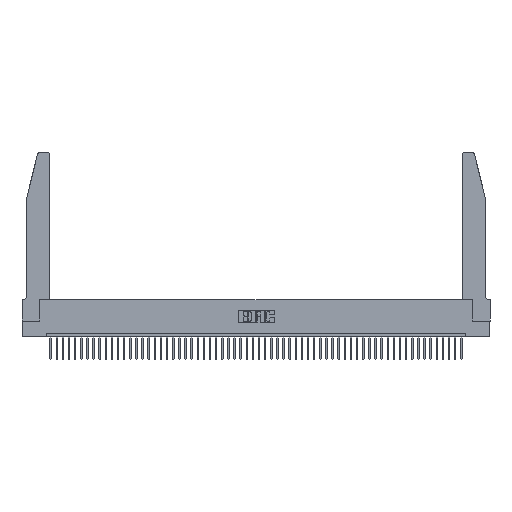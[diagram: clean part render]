
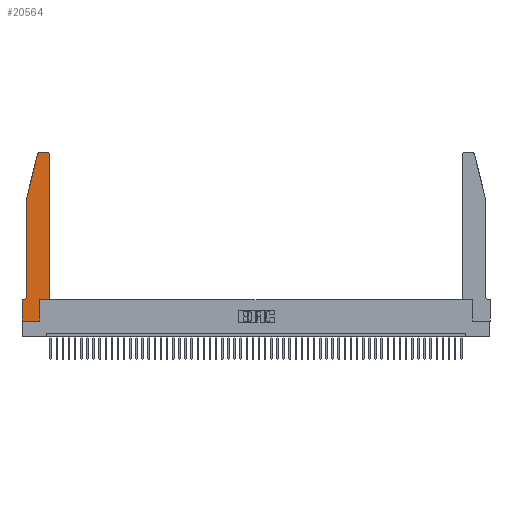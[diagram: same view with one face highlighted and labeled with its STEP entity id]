
A CAD part, top view. The second image highlights one B-rep face of the part: STEP entity #20564.
In plain terms, the highlighted planar face has unit normal (0, 0, 1).
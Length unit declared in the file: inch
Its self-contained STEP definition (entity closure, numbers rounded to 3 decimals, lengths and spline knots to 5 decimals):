
#170 = ORIENTED_EDGE ( 'NONE', *, *, #27050, .T. ) ;
#557 = CARTESIAN_POINT ( 'NONE',  ( 0.0055, 0.35, 0.37 ) ) ;
#560 = CARTESIAN_POINT ( 'NONE',  ( 0.4205, 2.75, 0.37 ) ) ;
#763 = VERTEX_POINT ( 'NONE', #13479 ) ;
#1389 = ORIENTED_EDGE ( 'NONE', *, *, #11748, .T. ) ;
#1840 = CARTESIAN_POINT ( 'NONE',  ( 0.0755, 2., 0.37 ) ) ;
#1872 = AXIS2_PLACEMENT_3D ( 'NONE', #17325, #6402, #38655 ) ;
#2724 = CARTESIAN_POINT ( 'NONE',  ( 0.0755, 0.42, 0.37 ) ) ;
#3187 = EDGE_CURVE ( 'NONE', #4844, #763, #23537, .T. ) ;
#3278 = EDGE_CURVE ( 'NONE', #38453, #35055, #41230, .T. ) ;
#4373 = VECTOR ( 'NONE', #25429, 39.37008 ) ;
#4844 = VERTEX_POINT ( 'NONE', #46409 ) ;
#5905 = DIRECTION ( 'NONE',  ( 0., 1., 0. ) ) ;
#6402 = DIRECTION ( 'NONE',  ( 0., 0., 1. ) ) ;
#6457 = VERTEX_POINT ( 'NONE', #557 ) ;
#6650 = LINE ( 'NONE', #36080, #19317 ) ;
#7045 = ORIENTED_EDGE ( 'NONE', *, *, #33911, .T. ) ;
#7117 = AXIS2_PLACEMENT_3D ( 'NONE', #15152, #44223, #43885 ) ;
#7120 = CARTESIAN_POINT ( 'NONE',  ( 0.2865, 0., 0.37 ) ) ;
#7476 = CARTESIAN_POINT ( 'NONE',  ( 0., 0., 0.37 ) ) ;
#8250 = LINE ( 'NONE', #39010, #17098 ) ;
#10651 = DIRECTION ( 'NONE',  ( 0., 1., 0. ) ) ;
#11029 = FACE_OUTER_BOUND ( 'NONE', #47378, .T. ) ;
#11257 = ORIENTED_EDGE ( 'NONE', *, *, #38534, .T. ) ;
#11748 = EDGE_CURVE ( 'NONE', #33758, #38453, #42578, .T. ) ;
#11949 = EDGE_CURVE ( 'NONE', #34345, #6457, #14689, .T. ) ;
#12480 = VERTEX_POINT ( 'NONE', #27450 ) ;
#12780 = LINE ( 'NONE', #49734, #30605 ) ;
#12926 = CARTESIAN_POINT ( 'NONE',  ( 0., 0., 0.37 ) ) ;
#13479 = CARTESIAN_POINT ( 'NONE',  ( 0.4505, 2.72, 0.37 ) ) ;
#13631 = VERTEX_POINT ( 'NONE', #42539 ) ;
#14689 = CIRCLE ( 'NONE', #44519, 0.07 ) ;
#15152 = CARTESIAN_POINT ( 'NONE',  ( 0., 0.35, 0.37 ) ) ;
#17098 = VECTOR ( 'NONE', #39556, 39.37008 ) ;
#17325 = CARTESIAN_POINT ( 'NONE',  ( 0.4205, 2.72, 0.37 ) ) ;
#17764 = CARTESIAN_POINT ( 'NONE',  ( 0.0755, 2., 0.37 ) ) ;
#19317 = VECTOR ( 'NONE', #28250, 39.37008 ) ;
#19671 = ORIENTED_EDGE ( 'NONE', *, *, #51198, .T. ) ;
#20564 = ADVANCED_FACE ( 'NONE', ( #11029 ), #27948, .T. ) ;
#22238 = CARTESIAN_POINT ( 'NONE',  ( 0.0755, 0.35, 0.37 ) ) ;
#22789 = ORIENTED_EDGE ( 'NONE', *, *, #3187, .T. ) ;
#23047 = VERTEX_POINT ( 'NONE', #48972 ) ;
#23537 = LINE ( 'NONE', #29133, #27998 ) ;
#23598 = DIRECTION ( 'NONE',  ( 1., 0., 0. ) ) ;
#25429 = DIRECTION ( 'NONE',  ( 0., -1., 0. ) ) ;
#25576 = CARTESIAN_POINT ( 'NONE',  ( 0., 0., 0.37 ) ) ;
#27050 = EDGE_CURVE ( 'NONE', #35055, #23047, #12780, .T. ) ;
#27436 = ORIENTED_EDGE ( 'NONE', *, *, #34682, .T. ) ;
#27450 = CARTESIAN_POINT ( 'NONE',  ( 0.284, 2.75, 0.37 ) ) ;
#27508 = CARTESIAN_POINT ( 'NONE',  ( 0.4505, 0.35, 0.37 ) ) ;
#27948 = PLANE ( 'NONE',  #7117 ) ;
#27998 = VECTOR ( 'NONE', #5905, 39.37008 ) ;
#28250 = DIRECTION ( 'NONE',  ( -0.239, -0.971, 0. ) ) ;
#29003 = LINE ( 'NONE', #22238, #30946 ) ;
#29133 = CARTESIAN_POINT ( 'NONE',  ( 0.4505, 0.35, 0.37 ) ) ;
#29560 = EDGE_CURVE ( 'NONE', #763, #35535, #46069, .T. ) ;
#30605 = VECTOR ( 'NONE', #10651, 39.37008 ) ;
#30667 = CARTESIAN_POINT ( 'NONE',  ( 0.0055, 0.42, 0.37 ) ) ;
#30946 = VECTOR ( 'NONE', #38593, 39.37008 ) ;
#32921 = CARTESIAN_POINT ( 'NONE',  ( 0., 0.35, 0.37 ) ) ;
#33758 = VERTEX_POINT ( 'NONE', #32921 ) ;
#33821 = ORIENTED_EDGE ( 'NONE', *, *, #36858, .T. ) ;
#33911 = EDGE_CURVE ( 'NONE', #23047, #4844, #50142, .T. ) ;
#34345 = VERTEX_POINT ( 'NONE', #2724 ) ;
#34682 = EDGE_CURVE ( 'NONE', #35535, #12480, #8250, .T. ) ;
#34852 = ORIENTED_EDGE ( 'NONE', *, *, #29560, .T. ) ;
#35055 = VERTEX_POINT ( 'NONE', #7120 ) ;
#35426 = EDGE_CURVE ( 'NONE', #35568, #34345, #36166, .T. ) ;
#35535 = VERTEX_POINT ( 'NONE', #560 ) ;
#35568 = VERTEX_POINT ( 'NONE', #1840 ) ;
#36080 = CARTESIAN_POINT ( 'NONE',  ( 0.0755, 2., 0.37 ) ) ;
#36166 = LINE ( 'NONE', #17764, #4373 ) ;
#36858 = EDGE_CURVE ( 'NONE', #13631, #35568, #6650, .T. ) ;
#37068 = ORIENTED_EDGE ( 'NONE', *, *, #35426, .T. ) ;
#37773 = ORIENTED_EDGE ( 'NONE', *, *, #3278, .T. ) ;
#38162 = VECTOR ( 'NONE', #39723, 39.37008 ) ;
#38453 = VERTEX_POINT ( 'NONE', #12926 ) ;
#38534 = EDGE_CURVE ( 'NONE', #12480, #13631, #47689, .T. ) ;
#38593 = DIRECTION ( 'NONE',  ( -1., 0., 0. ) ) ;
#38655 = DIRECTION ( 'NONE',  ( 1., 0., 0. ) ) ;
#38812 = DIRECTION ( 'NONE',  ( -1., 0., 0. ) ) ;
#39010 = CARTESIAN_POINT ( 'NONE',  ( 0.2605, 2.75, 0.37 ) ) ;
#39425 = DIRECTION ( 'NONE',  ( 1., 0., 0. ) ) ;
#39556 = DIRECTION ( 'NONE',  ( -1., 0., 0. ) ) ;
#39723 = DIRECTION ( 'NONE',  ( 1., 0., 0. ) ) ;
#40113 = CARTESIAN_POINT ( 'NONE',  ( 0.284, 2.72, 0.37 ) ) ;
#41230 = LINE ( 'NONE', #7476, #46287 ) ;
#42539 = CARTESIAN_POINT ( 'NONE',  ( 0.25487, 2.72718, 0.37 ) ) ;
#42578 = LINE ( 'NONE', #25576, #51478 ) ;
#43057 = DIRECTION ( 'NONE',  ( 0., 0., -1. ) ) ;
#43885 = DIRECTION ( 'NONE',  ( 1., 0., 0. ) ) ;
#44223 = DIRECTION ( 'NONE',  ( 0., 0., 1. ) ) ;
#44519 = AXIS2_PLACEMENT_3D ( 'NONE', #30667, #43057, #38812 ) ;
#45919 = AXIS2_PLACEMENT_3D ( 'NONE', #40113, #51629, #39425 ) ;
#46069 = CIRCLE ( 'NONE', #1872, 0.03 ) ;
#46287 = VECTOR ( 'NONE', #23598, 39.37008 ) ;
#46409 = CARTESIAN_POINT ( 'NONE',  ( 0.4505, 0.35, 0.37 ) ) ;
#47378 = EDGE_LOOP ( 'NONE', ( #27436, #11257, #33821, #37068, #50112, #19671, #1389, #37773, #170, #7045, #22789, #34852 ) ) ;
#47689 = CIRCLE ( 'NONE', #45919, 0.03 ) ;
#48972 = CARTESIAN_POINT ( 'NONE',  ( 0.2865, 0.35, 0.37 ) ) ;
#49734 = CARTESIAN_POINT ( 'NONE',  ( 0.2865, 0.35, 0.37 ) ) ;
#50112 = ORIENTED_EDGE ( 'NONE', *, *, #11949, .T. ) ;
#50142 = LINE ( 'NONE', #27508, #38162 ) ;
#50159 = DIRECTION ( 'NONE',  ( 0., -1., 0. ) ) ;
#51198 = EDGE_CURVE ( 'NONE', #6457, #33758, #29003, .T. ) ;
#51478 = VECTOR ( 'NONE', #50159, 39.37008 ) ;
#51629 = DIRECTION ( 'NONE',  ( 0., 0., 1. ) ) ;
